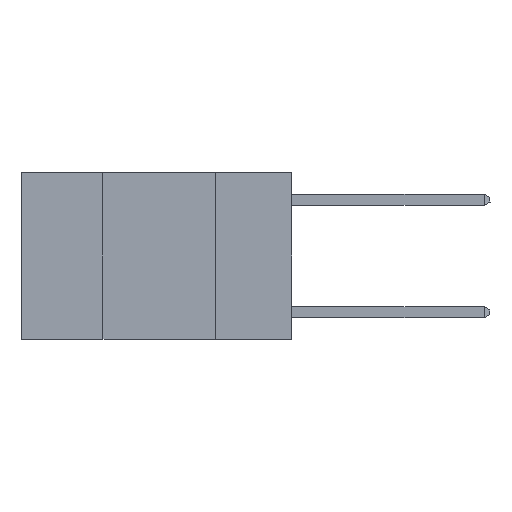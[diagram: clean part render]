
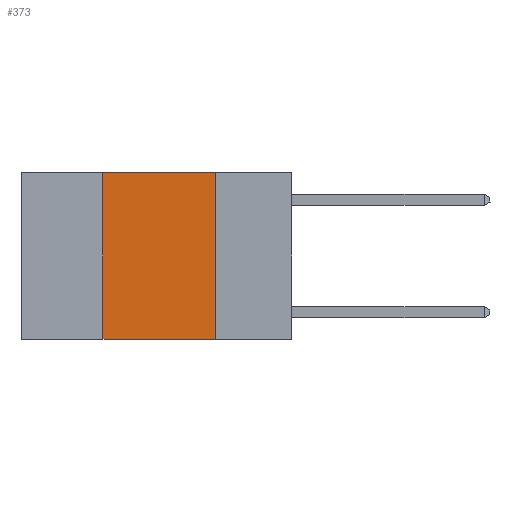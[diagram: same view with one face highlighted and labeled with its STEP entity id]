
A CAD part, left-side view. The second image highlights one B-rep face of the part: STEP entity #373.
In plain terms, the highlighted planar face has unit normal (-1, 0, 0).
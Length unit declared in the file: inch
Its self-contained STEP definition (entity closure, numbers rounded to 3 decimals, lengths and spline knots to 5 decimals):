
#331 = VERTEX_POINT ( 'NONE', #9373 ) ;
#373 = ADVANCED_FACE ( 'NONE', ( #21244 ), #1974, .F. ) ;
#731 = VECTOR ( 'NONE', #18751, 39.37008 ) ;
#1888 = CARTESIAN_POINT ( 'NONE',  ( 0., 0.6, 0. ) ) ;
#1974 = PLANE ( 'NONE',  #5901 ) ;
#2622 = VERTEX_POINT ( 'NONE', #8569 ) ;
#2967 = VERTEX_POINT ( 'NONE', #18832 ) ;
#3901 = DIRECTION ( 'NONE',  ( 0., 0., -1. ) ) ;
#5817 = CARTESIAN_POINT ( 'NONE',  ( 0., 0.42, 0. ) ) ;
#5901 = AXIS2_PLACEMENT_3D ( 'NONE', #1888, #15057, #3901 ) ;
#8104 = LINE ( 'NONE', #18236, #12451 ) ;
#8569 = CARTESIAN_POINT ( 'NONE',  ( 0., 0.42, -0.37 ) ) ;
#9089 = EDGE_CURVE ( 'NONE', #2622, #331, #10821, .T. ) ;
#9373 = CARTESIAN_POINT ( 'NONE',  ( 0., 0.17, -0.37 ) ) ;
#9401 = VECTOR ( 'NONE', #14858, 39.37008 ) ;
#9426 = EDGE_LOOP ( 'NONE', ( #9564, #9661, #9706, #9851 ) ) ;
#9564 = ORIENTED_EDGE ( 'NONE', *, *, #14082, .F. ) ;
#9661 = ORIENTED_EDGE ( 'NONE', *, *, #11463, .F. ) ;
#9706 = ORIENTED_EDGE ( 'NONE', *, *, #12844, .F. ) ;
#9851 = ORIENTED_EDGE ( 'NONE', *, *, #9089, .T. ) ;
#9874 = CARTESIAN_POINT ( 'NONE',  ( 0., 0.6, -0.37 ) ) ;
#10213 = VECTOR ( 'NONE', #22770, 39.37008 ) ;
#10821 = LINE ( 'NONE', #9874, #10213 ) ;
#11463 = EDGE_CURVE ( 'NONE', #2967, #22850, #14341, .T. ) ;
#12451 = VECTOR ( 'NONE', #12559, 39.37008 ) ;
#12559 = DIRECTION ( 'NONE',  ( 0., 0., -1. ) ) ;
#12844 = EDGE_CURVE ( 'NONE', #2622, #2967, #19464, .T. ) ;
#12999 = CARTESIAN_POINT ( 'NONE',  ( 0., 0.6, 0. ) ) ;
#14082 = EDGE_CURVE ( 'NONE', #22850, #331, #8104, .T. ) ;
#14341 = LINE ( 'NONE', #12999, #9401 ) ;
#14858 = DIRECTION ( 'NONE',  ( 0., -1., 0. ) ) ;
#15057 = DIRECTION ( 'NONE',  ( 1., 0., 0. ) ) ;
#18236 = CARTESIAN_POINT ( 'NONE',  ( 0., 0.17, 0. ) ) ;
#18751 = DIRECTION ( 'NONE',  ( 0., 0., 1. ) ) ;
#18832 = CARTESIAN_POINT ( 'NONE',  ( 0., 0.42, 0. ) ) ;
#19464 = LINE ( 'NONE', #5817, #731 ) ;
#20861 = CARTESIAN_POINT ( 'NONE',  ( 0., 0.17, 0. ) ) ;
#21244 = FACE_OUTER_BOUND ( 'NONE', #9426, .T. ) ;
#22770 = DIRECTION ( 'NONE',  ( 0., -1., 0. ) ) ;
#22850 = VERTEX_POINT ( 'NONE', #20861 ) ;
